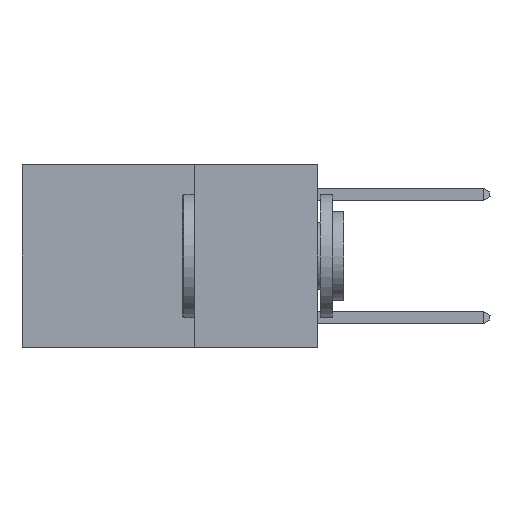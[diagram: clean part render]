
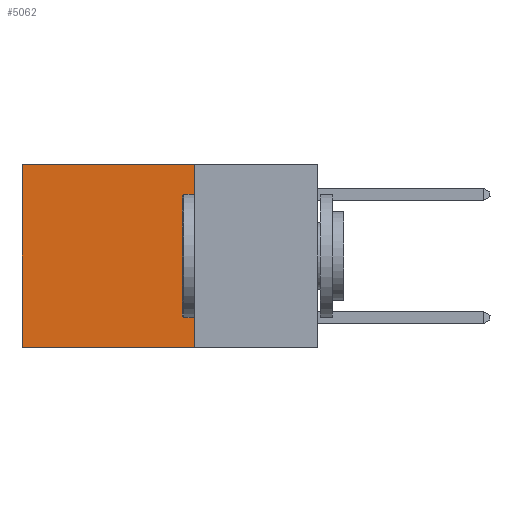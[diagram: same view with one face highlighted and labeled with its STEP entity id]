
A CAD part, left-side view. The second image highlights one B-rep face of the part: STEP entity #5062.
In plain terms, the highlighted planar face has unit normal (-1, 0, 0).
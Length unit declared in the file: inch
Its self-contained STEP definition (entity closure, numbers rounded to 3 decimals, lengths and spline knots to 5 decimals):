
#1373 = DIRECTION ( 'NONE',  ( 0., 0., -1. ) ) ;
#2240 = LINE ( 'NONE', #11280, #8790 ) ;
#2485 = EDGE_CURVE ( 'NONE', #3378, #7408, #5010, .T. ) ;
#2805 = CARTESIAN_POINT ( 'NONE',  ( 0.2625, 0.25, 0. ) ) ;
#3136 = VECTOR ( 'NONE', #7260, 39.37008 ) ;
#3256 = DIRECTION ( 'NONE',  ( 0., 0., -1. ) ) ;
#3378 = VERTEX_POINT ( 'NONE', #13900 ) ;
#3581 = PLANE ( 'NONE',  #11060 ) ;
#4197 = ORIENTED_EDGE ( 'NONE', *, *, #11579, .F. ) ;
#5010 = LINE ( 'NONE', #9562, #11732 ) ;
#5062 = ADVANCED_FACE ( 'NONE', ( #13580 ), #3581, .F. ) ;
#5620 = DIRECTION ( 'NONE',  ( 0., 0., -1. ) ) ;
#6602 = ORIENTED_EDGE ( 'NONE', *, *, #2485, .F. ) ;
#7260 = DIRECTION ( 'NONE',  ( 0., 1., 0. ) ) ;
#7408 = VERTEX_POINT ( 'NONE', #10326 ) ;
#7478 = VERTEX_POINT ( 'NONE', #9359 ) ;
#7933 = EDGE_CURVE ( 'NONE', #9027, #7478, #9534, .T. ) ;
#8092 = LINE ( 'NONE', #8320, #14030 ) ;
#8320 = CARTESIAN_POINT ( 'NONE',  ( 0.2625, 0.6, 0. ) ) ;
#8790 = VECTOR ( 'NONE', #3256, 39.37008 ) ;
#8839 = ORIENTED_EDGE ( 'NONE', *, *, #10546, .T. ) ;
#9027 = VERTEX_POINT ( 'NONE', #10087 ) ;
#9359 = CARTESIAN_POINT ( 'NONE',  ( 0.2625, 0.6, 0. ) ) ;
#9534 = LINE ( 'NONE', #2805, #3136 ) ;
#9562 = CARTESIAN_POINT ( 'NONE',  ( 0.2625, 0.25, -0.37 ) ) ;
#9821 = EDGE_LOOP ( 'NONE', ( #8839, #6602, #4197, #12391 ) ) ;
#10087 = CARTESIAN_POINT ( 'NONE',  ( 0.2625, 0.25, 0. ) ) ;
#10326 = CARTESIAN_POINT ( 'NONE',  ( 0.2625, 0.6, -0.37 ) ) ;
#10546 = EDGE_CURVE ( 'NONE', #7478, #7408, #8092, .T. ) ;
#11060 = AXIS2_PLACEMENT_3D ( 'NONE', #12558, #11461, #5620 ) ;
#11280 = CARTESIAN_POINT ( 'NONE',  ( 0.2625, 0.25, 0. ) ) ;
#11461 = DIRECTION ( 'NONE',  ( 1., 0., 0. ) ) ;
#11579 = EDGE_CURVE ( 'NONE', #9027, #3378, #2240, .T. ) ;
#11732 = VECTOR ( 'NONE', #14091, 39.37008 ) ;
#12391 = ORIENTED_EDGE ( 'NONE', *, *, #7933, .T. ) ;
#12558 = CARTESIAN_POINT ( 'NONE',  ( 0.2625, 0.25, 0. ) ) ;
#13580 = FACE_OUTER_BOUND ( 'NONE', #9821, .T. ) ;
#13900 = CARTESIAN_POINT ( 'NONE',  ( 0.2625, 0.25, -0.37 ) ) ;
#14030 = VECTOR ( 'NONE', #1373, 39.37008 ) ;
#14091 = DIRECTION ( 'NONE',  ( 0., 1., 0. ) ) ;
